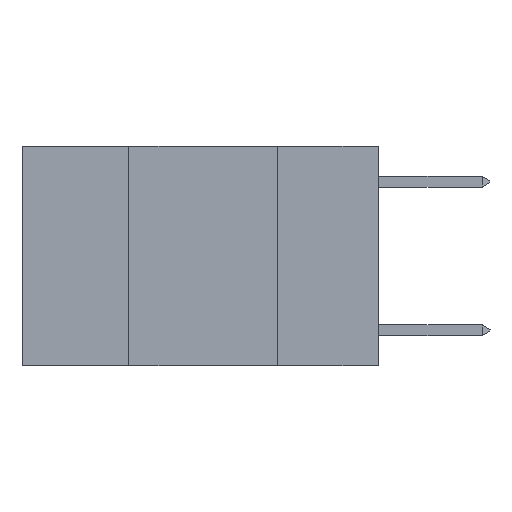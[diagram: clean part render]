
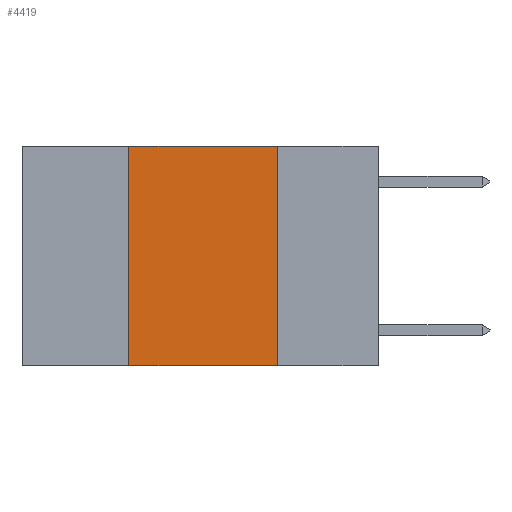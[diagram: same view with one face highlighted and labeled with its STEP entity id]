
A CAD part, left-side view. The second image highlights one B-rep face of the part: STEP entity #4419.
In plain terms, the highlighted planar face has unit normal (-1, 0, 0).
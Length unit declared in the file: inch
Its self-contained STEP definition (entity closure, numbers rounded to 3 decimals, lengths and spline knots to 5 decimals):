
#138 = DIRECTION ( 'NONE',  ( 0., 0., -1. ) ) ;
#376 = CARTESIAN_POINT ( 'NONE',  ( 0., 0.42, -0.37 ) ) ;
#533 = VERTEX_POINT ( 'NONE', #376 ) ;
#598 = EDGE_CURVE ( 'NONE', #4163, #6518, #9513, .T. ) ;
#627 = CARTESIAN_POINT ( 'NONE',  ( 0., 0.17, -0.37 ) ) ;
#764 = CARTESIAN_POINT ( 'NONE',  ( 0., 0.6, -0.37 ) ) ;
#908 = ORIENTED_EDGE ( 'NONE', *, *, #7657, .F. ) ;
#982 = EDGE_LOOP ( 'NONE', ( #6665, #4728, #908, #8533 ) ) ;
#1127 = AXIS2_PLACEMENT_3D ( 'NONE', #8982, #4753, #138 ) ;
#1316 = EDGE_CURVE ( 'NONE', #533, #6518, #8055, .T. ) ;
#1479 = VECTOR ( 'NONE', #3137, 39.37008 ) ;
#1757 = VERTEX_POINT ( 'NONE', #4175 ) ;
#2323 = FACE_OUTER_BOUND ( 'NONE', #982, .T. ) ;
#3137 = DIRECTION ( 'NONE',  ( 0., -1., 0. ) ) ;
#3618 = VECTOR ( 'NONE', #4677, 39.37008 ) ;
#4163 = VERTEX_POINT ( 'NONE', #6406 ) ;
#4175 = CARTESIAN_POINT ( 'NONE',  ( 0., 0.42, 0. ) ) ;
#4279 = CARTESIAN_POINT ( 'NONE',  ( 0., 0.42, 0. ) ) ;
#4419 = ADVANCED_FACE ( 'NONE', ( #2323 ), #8349, .F. ) ;
#4677 = DIRECTION ( 'NONE',  ( 0., 0., -1. ) ) ;
#4728 = ORIENTED_EDGE ( 'NONE', *, *, #8046, .F. ) ;
#4753 = DIRECTION ( 'NONE',  ( 1., 0., 0. ) ) ;
#4820 = VECTOR ( 'NONE', #9230, 39.37008 ) ;
#6154 = VECTOR ( 'NONE', #6921, 39.37008 ) ;
#6406 = CARTESIAN_POINT ( 'NONE',  ( 0., 0.17, 0. ) ) ;
#6518 = VERTEX_POINT ( 'NONE', #627 ) ;
#6665 = ORIENTED_EDGE ( 'NONE', *, *, #598, .F. ) ;
#6921 = DIRECTION ( 'NONE',  ( 0., -1., 0. ) ) ;
#6993 = LINE ( 'NONE', #4279, #4820 ) ;
#7657 = EDGE_CURVE ( 'NONE', #533, #1757, #6993, .T. ) ;
#7868 = CARTESIAN_POINT ( 'NONE',  ( 0., 0.17, 0. ) ) ;
#8046 = EDGE_CURVE ( 'NONE', #1757, #4163, #9004, .T. ) ;
#8055 = LINE ( 'NONE', #764, #6154 ) ;
#8248 = CARTESIAN_POINT ( 'NONE',  ( 0., 0.6, 0. ) ) ;
#8349 = PLANE ( 'NONE',  #1127 ) ;
#8533 = ORIENTED_EDGE ( 'NONE', *, *, #1316, .T. ) ;
#8982 = CARTESIAN_POINT ( 'NONE',  ( 0., 0.6, 0. ) ) ;
#9004 = LINE ( 'NONE', #8248, #1479 ) ;
#9230 = DIRECTION ( 'NONE',  ( 0., 0., 1. ) ) ;
#9513 = LINE ( 'NONE', #7868, #3618 ) ;
